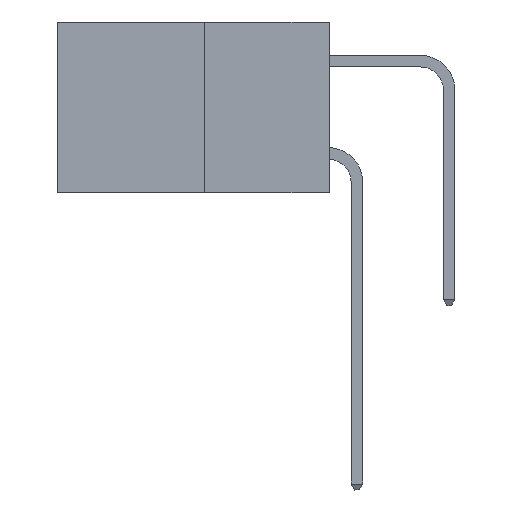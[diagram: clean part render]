
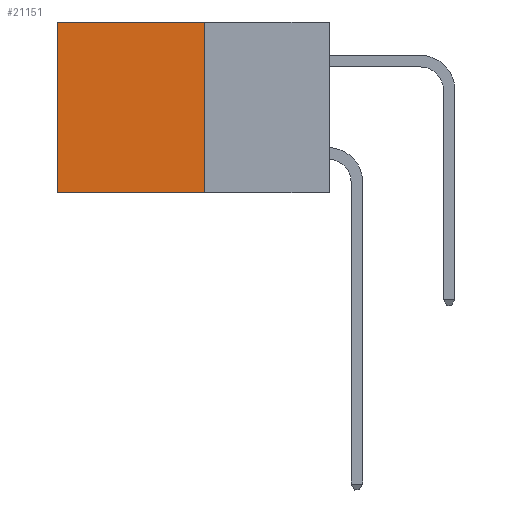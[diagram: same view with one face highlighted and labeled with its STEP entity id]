
A CAD part, left-side view. The second image highlights one B-rep face of the part: STEP entity #21151.
In plain terms, the highlighted planar face has unit normal (-1, 0, 0).
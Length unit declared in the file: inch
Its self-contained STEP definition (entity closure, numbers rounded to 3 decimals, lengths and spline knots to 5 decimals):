
#240 = ORIENTED_EDGE ( 'NONE', *, *, #2041, .F. ) ;
#1178 = EDGE_CURVE ( 'NONE', #26734, #11589, #9560, .T. ) ;
#1809 = FACE_OUTER_BOUND ( 'NONE', #11224, .T. ) ;
#1847 = CARTESIAN_POINT ( 'NONE',  ( 0.277, 0.27, 0. ) ) ;
#2041 = EDGE_CURVE ( 'NONE', #4738, #11589, #15022, .T. ) ;
#2497 = AXIS2_PLACEMENT_3D ( 'NONE', #2727, #17225, #4810 ) ;
#2727 = CARTESIAN_POINT ( 'NONE',  ( 0.277, 0.27, -0.37 ) ) ;
#3363 = LINE ( 'NONE', #7205, #19236 ) ;
#3890 = CARTESIAN_POINT ( 'NONE',  ( 0.277, 0.27, 0. ) ) ;
#4738 = VERTEX_POINT ( 'NONE', #16455 ) ;
#4810 = DIRECTION ( 'NONE',  ( 0., 0., -1. ) ) ;
#6153 = ORIENTED_EDGE ( 'NONE', *, *, #10149, .T. ) ;
#6664 = EDGE_CURVE ( 'NONE', #9500, #4738, #3363, .T. ) ;
#7205 = CARTESIAN_POINT ( 'NONE',  ( 0.277, 0.27, -0.37 ) ) ;
#7272 = DIRECTION ( 'NONE',  ( 0., 0., -1. ) ) ;
#8154 = CARTESIAN_POINT ( 'NONE',  ( 0.277, 0.59, 0. ) ) ;
#9500 = VERTEX_POINT ( 'NONE', #1847 ) ;
#9560 = LINE ( 'NONE', #23562, #19281 ) ;
#10149 = EDGE_CURVE ( 'NONE', #9500, #26734, #17800, .T. ) ;
#10577 = ORIENTED_EDGE ( 'NONE', *, *, #6664, .F. ) ;
#11224 = EDGE_LOOP ( 'NONE', ( #18307, #240, #10577, #6153 ) ) ;
#11589 = VERTEX_POINT ( 'NONE', #18998 ) ;
#13052 = PLANE ( 'NONE',  #2497 ) ;
#15022 = LINE ( 'NONE', #22735, #26696 ) ;
#16321 = DIRECTION ( 'NONE',  ( 0., 1., 0. ) ) ;
#16455 = CARTESIAN_POINT ( 'NONE',  ( 0.277, 0.27, -0.37 ) ) ;
#17225 = DIRECTION ( 'NONE',  ( 1., 0., 0. ) ) ;
#17800 = LINE ( 'NONE', #3890, #22668 ) ;
#18307 = ORIENTED_EDGE ( 'NONE', *, *, #1178, .T. ) ;
#18998 = CARTESIAN_POINT ( 'NONE',  ( 0.277, 0.59, -0.37 ) ) ;
#19236 = VECTOR ( 'NONE', #7272, 39.37008 ) ;
#19281 = VECTOR ( 'NONE', #22844, 39.37008 ) ;
#21151 = ADVANCED_FACE ( 'NONE', ( #1809 ), #13052, .F. ) ;
#21485 = DIRECTION ( 'NONE',  ( 0., 1., 0. ) ) ;
#22668 = VECTOR ( 'NONE', #16321, 39.37008 ) ;
#22735 = CARTESIAN_POINT ( 'NONE',  ( 0.277, 0.27, -0.37 ) ) ;
#22844 = DIRECTION ( 'NONE',  ( 0., 0., -1. ) ) ;
#23562 = CARTESIAN_POINT ( 'NONE',  ( 0.277, 0.59, -0.37 ) ) ;
#26696 = VECTOR ( 'NONE', #21485, 39.37008 ) ;
#26734 = VERTEX_POINT ( 'NONE', #8154 ) ;
